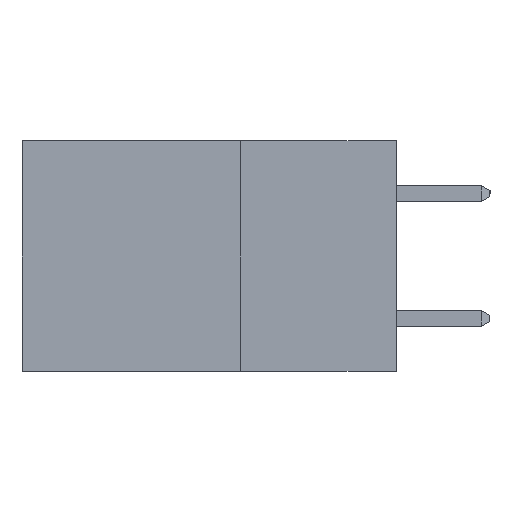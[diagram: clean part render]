
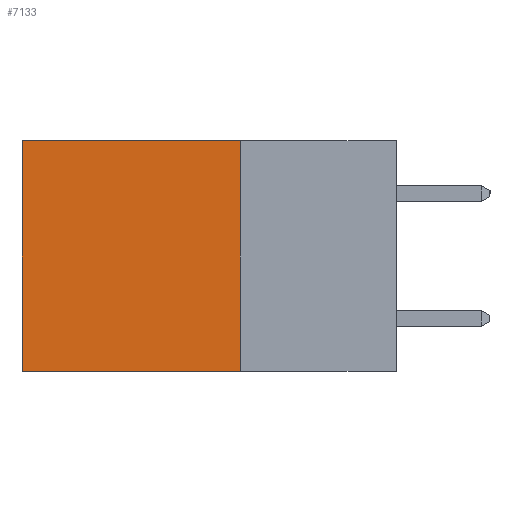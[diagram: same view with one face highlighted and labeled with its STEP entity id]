
A CAD part, left-side view. The second image highlights one B-rep face of the part: STEP entity #7133.
In plain terms, the highlighted planar face has unit normal (-1, 0, 0).
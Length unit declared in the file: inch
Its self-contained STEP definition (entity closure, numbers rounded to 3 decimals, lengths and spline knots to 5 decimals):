
#464 = DIRECTION ( 'NONE',  ( 0., 1., 0. ) ) ;
#507 = CARTESIAN_POINT ( 'NONE',  ( 0.2615, 0.6, 0. ) ) ;
#835 = LINE ( 'NONE', #3799, #5787 ) ;
#1506 = DIRECTION ( 'NONE',  ( 0., 0., -1. ) ) ;
#1923 = LINE ( 'NONE', #10142, #8246 ) ;
#2581 = EDGE_CURVE ( 'NONE', #9297, #3006, #1923, .T. ) ;
#3006 = VERTEX_POINT ( 'NONE', #507 ) ;
#3799 = CARTESIAN_POINT ( 'NONE',  ( 0.2615, 0.6, -0.37 ) ) ;
#3803 = ORIENTED_EDGE ( 'NONE', *, *, #7979, .T. ) ;
#4122 = PLANE ( 'NONE',  #16206 ) ;
#4269 = VERTEX_POINT ( 'NONE', #8974 ) ;
#5787 = VECTOR ( 'NONE', #13368, 39.37008 ) ;
#6597 = ORIENTED_EDGE ( 'NONE', *, *, #10828, .F. ) ;
#6600 = DIRECTION ( 'NONE',  ( 0., 1., 0. ) ) ;
#7133 = ADVANCED_FACE ( 'NONE', ( #10997 ), #4122, .F. ) ;
#7277 = CARTESIAN_POINT ( 'NONE',  ( 0.2615, 0.25, -0.37 ) ) ;
#7979 = EDGE_CURVE ( 'NONE', #3006, #4269, #835, .T. ) ;
#8246 = VECTOR ( 'NONE', #464, 39.37008 ) ;
#8341 = ORIENTED_EDGE ( 'NONE', *, *, #2581, .T. ) ;
#8365 = CARTESIAN_POINT ( 'NONE',  ( 0.2615, 0.25, -0.37 ) ) ;
#8974 = CARTESIAN_POINT ( 'NONE',  ( 0.2615, 0.6, -0.37 ) ) ;
#9226 = VECTOR ( 'NONE', #6600, 39.37008 ) ;
#9297 = VERTEX_POINT ( 'NONE', #11506 ) ;
#9654 = DIRECTION ( 'NONE',  ( 1., 0., 0. ) ) ;
#10142 = CARTESIAN_POINT ( 'NONE',  ( 0.2615, 0.25, 0. ) ) ;
#10828 = EDGE_CURVE ( 'NONE', #15064, #4269, #14814, .T. ) ;
#10997 = FACE_OUTER_BOUND ( 'NONE', #13471, .T. ) ;
#11506 = CARTESIAN_POINT ( 'NONE',  ( 0.2615, 0.25, 0. ) ) ;
#13368 = DIRECTION ( 'NONE',  ( 0., 0., -1. ) ) ;
#13471 = EDGE_LOOP ( 'NONE', ( #3803, #6597, #15934, #8341 ) ) ;
#13542 = CARTESIAN_POINT ( 'NONE',  ( 0.2615, 0.25, -0.37 ) ) ;
#14814 = LINE ( 'NONE', #13542, #9226 ) ;
#15064 = VERTEX_POINT ( 'NONE', #7277 ) ;
#15394 = VECTOR ( 'NONE', #15932, 39.37008 ) ;
#15932 = DIRECTION ( 'NONE',  ( 0., 0., -1. ) ) ;
#15934 = ORIENTED_EDGE ( 'NONE', *, *, #17358, .F. ) ;
#16206 = AXIS2_PLACEMENT_3D ( 'NONE', #8365, #9654, #1506 ) ;
#17269 = CARTESIAN_POINT ( 'NONE',  ( 0.2615, 0.25, -0.37 ) ) ;
#17358 = EDGE_CURVE ( 'NONE', #9297, #15064, #17453, .T. ) ;
#17453 = LINE ( 'NONE', #17269, #15394 ) ;
